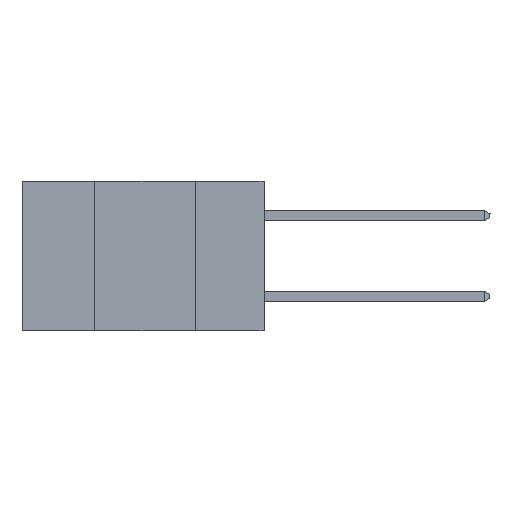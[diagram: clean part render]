
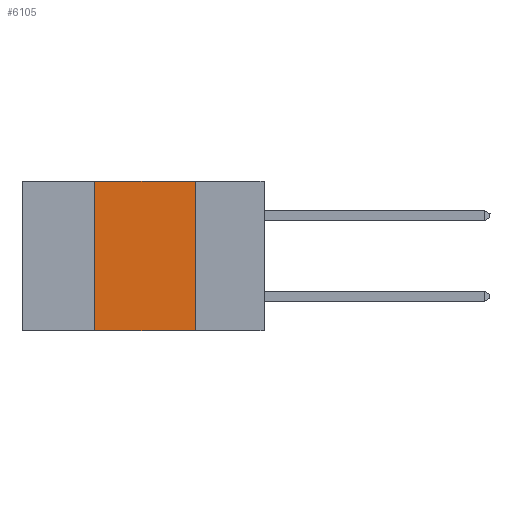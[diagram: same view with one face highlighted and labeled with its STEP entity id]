
A CAD part, left-side view. The second image highlights one B-rep face of the part: STEP entity #6105.
In plain terms, the highlighted planar face has unit normal (-1, 0, 0).
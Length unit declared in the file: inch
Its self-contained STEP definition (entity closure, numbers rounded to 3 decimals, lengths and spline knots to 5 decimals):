
#539 = LINE ( 'NONE', #25444, #28629 ) ;
#799 = VERTEX_POINT ( 'NONE', #18185 ) ;
#1608 = VECTOR ( 'NONE', #26519, 39.37008 ) ;
#2052 = EDGE_CURVE ( 'NONE', #21407, #8784, #27842, .T. ) ;
#2847 = DIRECTION ( 'NONE',  ( 1., 0., 0. ) ) ;
#3524 = ORIENTED_EDGE ( 'NONE', *, *, #19049, .F. ) ;
#4464 = LINE ( 'NONE', #11910, #15746 ) ;
#5233 = DIRECTION ( 'NONE',  ( 0., 0., -1. ) ) ;
#6105 = ADVANCED_FACE ( 'NONE', ( #26893 ), #26260, .F. ) ;
#8784 = VERTEX_POINT ( 'NONE', #26191 ) ;
#9441 = DIRECTION ( 'NONE',  ( 0., -1., 0. ) ) ;
#9717 = ORIENTED_EDGE ( 'NONE', *, *, #13500, .F. ) ;
#11910 = CARTESIAN_POINT ( 'NONE',  ( 0., 0.17, 0. ) ) ;
#12473 = EDGE_LOOP ( 'NONE', ( #3524, #9717, #21899, #29133 ) ) ;
#12674 = CARTESIAN_POINT ( 'NONE',  ( 0., 0.6, -0.37 ) ) ;
#13067 = AXIS2_PLACEMENT_3D ( 'NONE', #18920, #2847, #5233 ) ;
#13500 = EDGE_CURVE ( 'NONE', #799, #16831, #539, .T. ) ;
#14507 = CARTESIAN_POINT ( 'NONE',  ( 0., 0.42, 0. ) ) ;
#14740 = VECTOR ( 'NONE', #28785, 39.37008 ) ;
#15746 = VECTOR ( 'NONE', #23542, 39.37008 ) ;
#16831 = VERTEX_POINT ( 'NONE', #21770 ) ;
#17828 = EDGE_CURVE ( 'NONE', #21407, #799, #23878, .T. ) ;
#18185 = CARTESIAN_POINT ( 'NONE',  ( 0., 0.42, 0. ) ) ;
#18920 = CARTESIAN_POINT ( 'NONE',  ( 0., 0.6, 0. ) ) ;
#19049 = EDGE_CURVE ( 'NONE', #16831, #8784, #4464, .T. ) ;
#21407 = VERTEX_POINT ( 'NONE', #21721 ) ;
#21721 = CARTESIAN_POINT ( 'NONE',  ( 0., 0.42, -0.37 ) ) ;
#21770 = CARTESIAN_POINT ( 'NONE',  ( 0., 0.17, 0. ) ) ;
#21899 = ORIENTED_EDGE ( 'NONE', *, *, #17828, .F. ) ;
#23542 = DIRECTION ( 'NONE',  ( 0., 0., -1. ) ) ;
#23878 = LINE ( 'NONE', #14507, #1608 ) ;
#25444 = CARTESIAN_POINT ( 'NONE',  ( 0., 0.6, 0. ) ) ;
#26191 = CARTESIAN_POINT ( 'NONE',  ( 0., 0.17, -0.37 ) ) ;
#26260 = PLANE ( 'NONE',  #13067 ) ;
#26519 = DIRECTION ( 'NONE',  ( 0., 0., 1. ) ) ;
#26893 = FACE_OUTER_BOUND ( 'NONE', #12473, .T. ) ;
#27842 = LINE ( 'NONE', #12674, #14740 ) ;
#28629 = VECTOR ( 'NONE', #9441, 39.37008 ) ;
#28785 = DIRECTION ( 'NONE',  ( 0., -1., 0. ) ) ;
#29133 = ORIENTED_EDGE ( 'NONE', *, *, #2052, .T. ) ;
